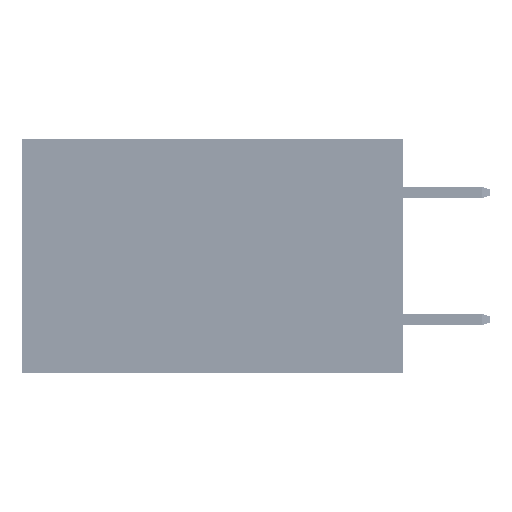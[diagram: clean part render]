
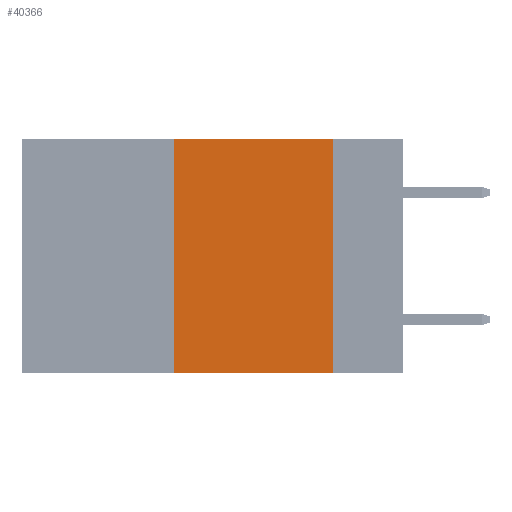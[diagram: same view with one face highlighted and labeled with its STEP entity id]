
A CAD part, left-side view. The second image highlights one B-rep face of the part: STEP entity #40366.
In plain terms, the highlighted planar face has unit normal (-1, 0, 0).
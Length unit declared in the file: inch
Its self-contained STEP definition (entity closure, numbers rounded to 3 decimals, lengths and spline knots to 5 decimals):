
#536 = EDGE_CURVE ( 'NONE', #33823, #6659, #28939, .T. ) ;
#2844 = EDGE_CURVE ( 'NONE', #33823, #30318, #43403, .T. ) ;
#3381 = ORIENTED_EDGE ( 'NONE', *, *, #31999, .F. ) ;
#6009 = VECTOR ( 'NONE', #27788, 39.37008 ) ;
#6659 = VERTEX_POINT ( 'NONE', #24669 ) ;
#7338 = ORIENTED_EDGE ( 'NONE', *, *, #2844, .T. ) ;
#9479 = DIRECTION ( 'NONE',  ( 0., 0., 1. ) ) ;
#9957 = DIRECTION ( 'NONE',  ( 0., -1., 0. ) ) ;
#11837 = AXIS2_PLACEMENT_3D ( 'NONE', #28844, #40788, #48606 ) ;
#16160 = LINE ( 'NONE', #48355, #45767 ) ;
#17107 = CARTESIAN_POINT ( 'NONE',  ( 0., 0.36, -0.37 ) ) ;
#21399 = ORIENTED_EDGE ( 'NONE', *, *, #536, .F. ) ;
#24669 = CARTESIAN_POINT ( 'NONE',  ( 0., 0.36, 0. ) ) ;
#25205 = PLANE ( 'NONE',  #11837 ) ;
#26833 = CARTESIAN_POINT ( 'NONE',  ( 0., 0.11, 0. ) ) ;
#27265 = CARTESIAN_POINT ( 'NONE',  ( 0., 0.6, -0.37 ) ) ;
#27788 = DIRECTION ( 'NONE',  ( 0., -1., 0. ) ) ;
#28326 = FACE_OUTER_BOUND ( 'NONE', #48505, .T. ) ;
#28844 = CARTESIAN_POINT ( 'NONE',  ( 0., 0.6, 0. ) ) ;
#28939 = LINE ( 'NONE', #44796, #31394 ) ;
#30318 = VERTEX_POINT ( 'NONE', #49709 ) ;
#31331 = VERTEX_POINT ( 'NONE', #26833 ) ;
#31394 = VECTOR ( 'NONE', #9479, 39.37008 ) ;
#31999 = EDGE_CURVE ( 'NONE', #31331, #30318, #16160, .T. ) ;
#32493 = DIRECTION ( 'NONE',  ( 0., 0., -1. ) ) ;
#33823 = VERTEX_POINT ( 'NONE', #17107 ) ;
#37458 = LINE ( 'NONE', #45530, #50842 ) ;
#40209 = EDGE_CURVE ( 'NONE', #6659, #31331, #37458, .T. ) ;
#40366 = ADVANCED_FACE ( 'NONE', ( #28326 ), #25205, .F. ) ;
#40788 = DIRECTION ( 'NONE',  ( 1., 0., 0. ) ) ;
#43403 = LINE ( 'NONE', #27265, #6009 ) ;
#44796 = CARTESIAN_POINT ( 'NONE',  ( 0., 0.36, 0. ) ) ;
#45530 = CARTESIAN_POINT ( 'NONE',  ( 0., 0.6, 0. ) ) ;
#45767 = VECTOR ( 'NONE', #32493, 39.37008 ) ;
#46506 = ORIENTED_EDGE ( 'NONE', *, *, #40209, .F. ) ;
#48355 = CARTESIAN_POINT ( 'NONE',  ( 0., 0.11, 0. ) ) ;
#48505 = EDGE_LOOP ( 'NONE', ( #3381, #46506, #21399, #7338 ) ) ;
#48606 = DIRECTION ( 'NONE',  ( 0., 0., -1. ) ) ;
#49709 = CARTESIAN_POINT ( 'NONE',  ( 0., 0.11, -0.37 ) ) ;
#50842 = VECTOR ( 'NONE', #9957, 39.37008 ) ;
